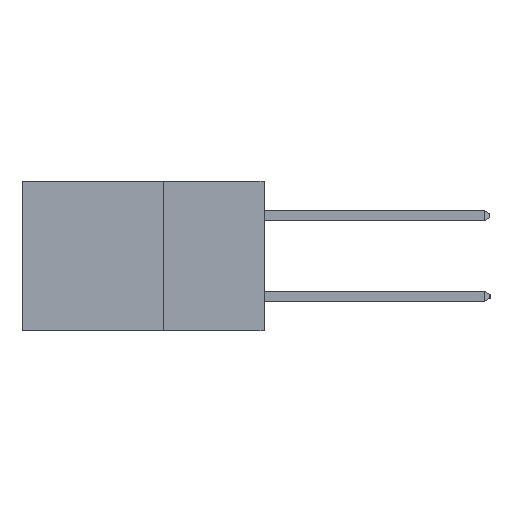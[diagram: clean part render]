
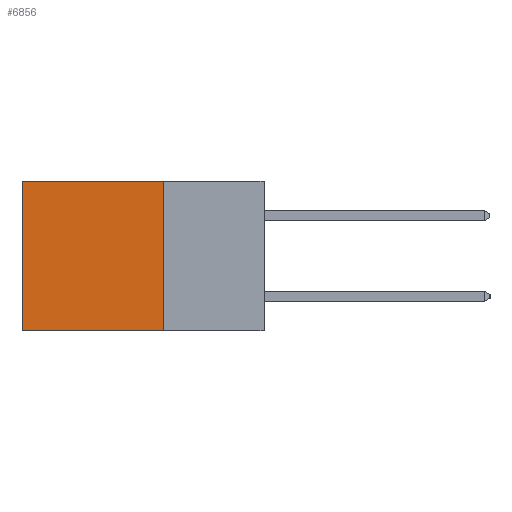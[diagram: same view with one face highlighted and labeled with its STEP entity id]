
A CAD part, left-side view. The second image highlights one B-rep face of the part: STEP entity #6856.
In plain terms, the highlighted planar face has unit normal (-1, 0, 0).
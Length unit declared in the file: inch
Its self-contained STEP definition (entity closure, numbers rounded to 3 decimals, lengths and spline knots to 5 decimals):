
#240 = VERTEX_POINT ( 'NONE', #10583 ) ;
#354 = ORIENTED_EDGE ( 'NONE', *, *, #9047, .F. ) ;
#480 = DIRECTION ( 'NONE',  ( 0., 0., -1. ) ) ;
#1077 = DIRECTION ( 'NONE',  ( 0., 0., -1. ) ) ;
#1401 = EDGE_CURVE ( 'NONE', #7447, #240, #9612, .T. ) ;
#1648 = CARTESIAN_POINT ( 'NONE',  ( 0.2615, 0.6, -0.37 ) ) ;
#2228 = CARTESIAN_POINT ( 'NONE',  ( 0.2615, 0.25, -0.37 ) ) ;
#3242 = CARTESIAN_POINT ( 'NONE',  ( 0.2615, 0.25, -0.37 ) ) ;
#3643 = EDGE_LOOP ( 'NONE', ( #13375, #8146, #354, #5431 ) ) ;
#4022 = VECTOR ( 'NONE', #7805, 39.37008 ) ;
#4269 = LINE ( 'NONE', #7392, #9833 ) ;
#4809 = DIRECTION ( 'NONE',  ( 0., 1., 0. ) ) ;
#5431 = ORIENTED_EDGE ( 'NONE', *, *, #1401, .T. ) ;
#5511 = FACE_OUTER_BOUND ( 'NONE', #3643, .T. ) ;
#5604 = DIRECTION ( 'NONE',  ( 1., 0., 0. ) ) ;
#6002 = AXIS2_PLACEMENT_3D ( 'NONE', #2228, #5604, #13214 ) ;
#6856 = ADVANCED_FACE ( 'NONE', ( #5511 ), #12161, .F. ) ;
#6918 = EDGE_CURVE ( 'NONE', #240, #8083, #8152, .T. ) ;
#7392 = CARTESIAN_POINT ( 'NONE',  ( 0.2615, 0.25, -0.37 ) ) ;
#7447 = VERTEX_POINT ( 'NONE', #10786 ) ;
#7805 = DIRECTION ( 'NONE',  ( 0., 1., 0. ) ) ;
#7812 = VECTOR ( 'NONE', #1077, 39.37008 ) ;
#7915 = CARTESIAN_POINT ( 'NONE',  ( 0.2615, 0.25, 0. ) ) ;
#7921 = EDGE_CURVE ( 'NONE', #8394, #8083, #12997, .T. ) ;
#8083 = VERTEX_POINT ( 'NONE', #1648 ) ;
#8146 = ORIENTED_EDGE ( 'NONE', *, *, #7921, .F. ) ;
#8152 = LINE ( 'NONE', #14246, #7812 ) ;
#8394 = VERTEX_POINT ( 'NONE', #3242 ) ;
#9047 = EDGE_CURVE ( 'NONE', #7447, #8394, #4269, .T. ) ;
#9612 = LINE ( 'NONE', #7915, #4022 ) ;
#9833 = VECTOR ( 'NONE', #480, 39.37008 ) ;
#10583 = CARTESIAN_POINT ( 'NONE',  ( 0.2615, 0.6, 0. ) ) ;
#10786 = CARTESIAN_POINT ( 'NONE',  ( 0.2615, 0.25, 0. ) ) ;
#12161 = PLANE ( 'NONE',  #6002 ) ;
#12474 = CARTESIAN_POINT ( 'NONE',  ( 0.2615, 0.25, -0.37 ) ) ;
#12672 = VECTOR ( 'NONE', #4809, 39.37008 ) ;
#12997 = LINE ( 'NONE', #12474, #12672 ) ;
#13214 = DIRECTION ( 'NONE',  ( 0., 0., -1. ) ) ;
#13375 = ORIENTED_EDGE ( 'NONE', *, *, #6918, .T. ) ;
#14246 = CARTESIAN_POINT ( 'NONE',  ( 0.2615, 0.6, -0.37 ) ) ;
